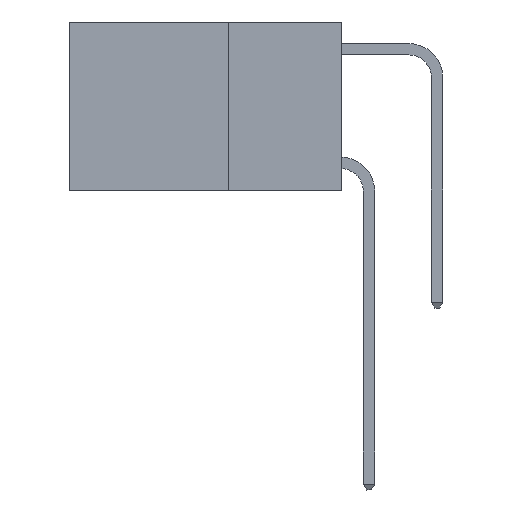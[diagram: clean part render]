
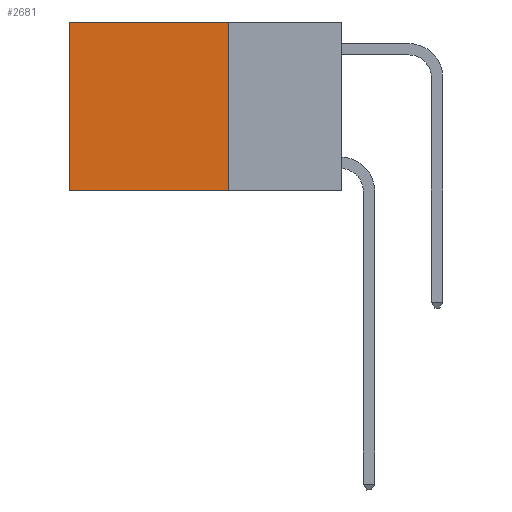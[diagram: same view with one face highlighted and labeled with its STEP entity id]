
A CAD part, left-side view. The second image highlights one B-rep face of the part: STEP entity #2681.
In plain terms, the highlighted planar face has unit normal (-1, 0, 0).
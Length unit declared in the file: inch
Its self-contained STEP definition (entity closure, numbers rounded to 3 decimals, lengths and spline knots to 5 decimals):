
#264 = AXIS2_PLACEMENT_3D ( 'NONE', #2660, #2736, #9389 ) ;
#615 = CARTESIAN_POINT ( 'NONE',  ( 0.2625, 0.25, -0.37 ) ) ;
#804 = CARTESIAN_POINT ( 'NONE',  ( 0.2625, 0.25, 0. ) ) ;
#844 = LINE ( 'NONE', #13135, #13466 ) ;
#1111 = CARTESIAN_POINT ( 'NONE',  ( 0.2625, 0.25, 0. ) ) ;
#1641 = VERTEX_POINT ( 'NONE', #615 ) ;
#2039 = LINE ( 'NONE', #804, #5311 ) ;
#2053 = EDGE_CURVE ( 'NONE', #1641, #9239, #2880, .T. ) ;
#2444 = PLANE ( 'NONE',  #264 ) ;
#2660 = CARTESIAN_POINT ( 'NONE',  ( 0.2625, 0.25, 0. ) ) ;
#2681 = ADVANCED_FACE ( 'NONE', ( #10287 ), #2444, .F. ) ;
#2736 = DIRECTION ( 'NONE',  ( 1., 0., 0. ) ) ;
#2880 = LINE ( 'NONE', #11686, #9074 ) ;
#3299 = ORIENTED_EDGE ( 'NONE', *, *, #7801, .T. ) ;
#3646 = VERTEX_POINT ( 'NONE', #1111 ) ;
#4292 = DIRECTION ( 'NONE',  ( 0., 0., -1. ) ) ;
#5186 = DIRECTION ( 'NONE',  ( 0., 1., 0. ) ) ;
#5246 = EDGE_CURVE ( 'NONE', #3646, #1641, #2039, .T. ) ;
#5311 = VECTOR ( 'NONE', #4292, 39.37008 ) ;
#7801 = EDGE_CURVE ( 'NONE', #3646, #10234, #8366, .T. ) ;
#8366 = LINE ( 'NONE', #9292, #10437 ) ;
#8435 = DIRECTION ( 'NONE',  ( 0., 1., 0. ) ) ;
#8631 = ORIENTED_EDGE ( 'NONE', *, *, #5246, .F. ) ;
#9074 = VECTOR ( 'NONE', #5186, 39.37008 ) ;
#9239 = VERTEX_POINT ( 'NONE', #11872 ) ;
#9288 = CARTESIAN_POINT ( 'NONE',  ( 0.2625, 0.6, 0. ) ) ;
#9292 = CARTESIAN_POINT ( 'NONE',  ( 0.2625, 0.25, 0. ) ) ;
#9322 = EDGE_LOOP ( 'NONE', ( #11186, #12241, #8631, #3299 ) ) ;
#9389 = DIRECTION ( 'NONE',  ( 0., 0., -1. ) ) ;
#9523 = EDGE_CURVE ( 'NONE', #10234, #9239, #844, .T. ) ;
#10234 = VERTEX_POINT ( 'NONE', #9288 ) ;
#10287 = FACE_OUTER_BOUND ( 'NONE', #9322, .T. ) ;
#10437 = VECTOR ( 'NONE', #8435, 39.37008 ) ;
#11186 = ORIENTED_EDGE ( 'NONE', *, *, #9523, .T. ) ;
#11686 = CARTESIAN_POINT ( 'NONE',  ( 0.2625, 0.25, -0.37 ) ) ;
#11872 = CARTESIAN_POINT ( 'NONE',  ( 0.2625, 0.6, -0.37 ) ) ;
#12241 = ORIENTED_EDGE ( 'NONE', *, *, #2053, .F. ) ;
#12854 = DIRECTION ( 'NONE',  ( 0., 0., -1. ) ) ;
#13135 = CARTESIAN_POINT ( 'NONE',  ( 0.2625, 0.6, 0. ) ) ;
#13466 = VECTOR ( 'NONE', #12854, 39.37008 ) ;
